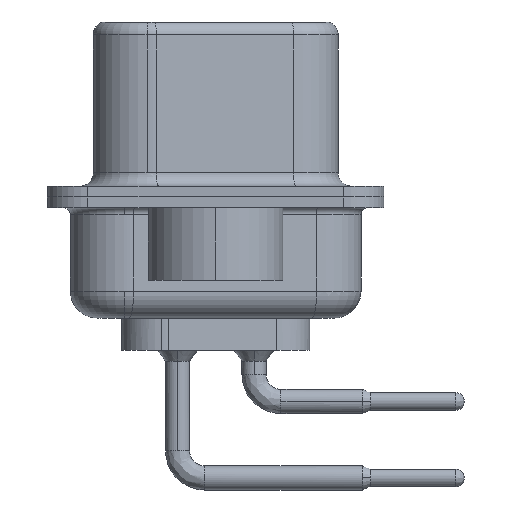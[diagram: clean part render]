
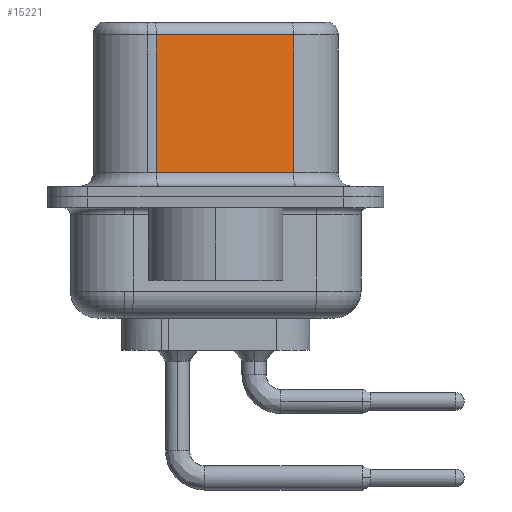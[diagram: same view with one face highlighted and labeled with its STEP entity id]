
A CAD part, left-side view. The second image highlights one B-rep face of the part: STEP entity #15221.
In plain terms, the highlighted planar face has unit normal (-0.985, -0.174, 0).
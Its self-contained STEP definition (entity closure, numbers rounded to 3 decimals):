
#180 = EDGE_CURVE ( 'NONE', #8894, #14508, #8443, .T. ) ;
#233 = DIRECTION ( 'NONE',  ( 0., 0., -1. ) ) ;
#1543 = ORIENTED_EDGE ( 'NONE', *, *, #8638, .T. ) ;
#1606 = EDGE_LOOP ( 'NONE', ( #16887, #12089, #1543, #5080 ) ) ;
#3811 = LINE ( 'NONE', #17249, #11841 ) ;
#4176 = DIRECTION ( 'NONE',  ( 0., 0., -1. ) ) ;
#4678 = CARTESIAN_POINT ( 'NONE',  ( 4.555, -2.897, 6.02 ) ) ;
#5080 = ORIENTED_EDGE ( 'NONE', *, *, #180, .T. ) ;
#6333 = DIRECTION ( 'NONE',  ( -0.174, 0.985, 0. ) ) ;
#7077 = CARTESIAN_POINT ( 'NONE',  ( 4.555, -2.897, 0.9 ) ) ;
#7120 = CARTESIAN_POINT ( 'NONE',  ( 4.555, -2.897, 6.52 ) ) ;
#7264 = FACE_OUTER_BOUND ( 'NONE', #1606, .T. ) ;
#8443 = LINE ( 'NONE', #22059, #11897 ) ;
#8638 = EDGE_CURVE ( 'NONE', #18784, #8894, #19244, .T. ) ;
#8842 = DIRECTION ( 'NONE',  ( 0.985, 0.174, 0. ) ) ;
#8894 = VERTEX_POINT ( 'NONE', #10180 ) ;
#9284 = CARTESIAN_POINT ( 'NONE',  ( 3.655, 2.203, 6.52 ) ) ;
#9553 = EDGE_CURVE ( 'NONE', #11536, #18784, #11789, .T. ) ;
#10180 = CARTESIAN_POINT ( 'NONE',  ( 3.655, 2.203, 0.9 ) ) ;
#10235 = VECTOR ( 'NONE', #4176, 1000. ) ;
#11536 = VERTEX_POINT ( 'NONE', #12298 ) ;
#11789 = LINE ( 'NONE', #4678, #20302 ) ;
#11841 = VECTOR ( 'NONE', #233, 1000. ) ;
#11897 = VECTOR ( 'NONE', #18344, 1000. ) ;
#12089 = ORIENTED_EDGE ( 'NONE', *, *, #9553, .T. ) ;
#12298 = CARTESIAN_POINT ( 'NONE',  ( 4.555, -2.897, 6.02 ) ) ;
#13858 = PLANE ( 'NONE',  #21511 ) ;
#14508 = VERTEX_POINT ( 'NONE', #7077 ) ;
#15221 = ADVANCED_FACE ( 'NONE', ( #7264 ), #13858, .F. ) ;
#16887 = ORIENTED_EDGE ( 'NONE', *, *, #18919, .F. ) ;
#17249 = CARTESIAN_POINT ( 'NONE',  ( 4.555, -2.897, 6.52 ) ) ;
#18344 = DIRECTION ( 'NONE',  ( 0.174, -0.985, 0. ) ) ;
#18784 = VERTEX_POINT ( 'NONE', #22076 ) ;
#18919 = EDGE_CURVE ( 'NONE', #11536, #14508, #3811, .T. ) ;
#19244 = LINE ( 'NONE', #9284, #10235 ) ;
#20302 = VECTOR ( 'NONE', #6333, 1000. ) ;
#20746 = DIRECTION ( 'NONE',  ( -0.174, 0.985, 0. ) ) ;
#21511 = AXIS2_PLACEMENT_3D ( 'NONE', #7120, #8842, #20746 ) ;
#22059 = CARTESIAN_POINT ( 'NONE',  ( 4.555, -2.897, 0.9 ) ) ;
#22076 = CARTESIAN_POINT ( 'NONE',  ( 3.655, 2.203, 6.02 ) ) ;
